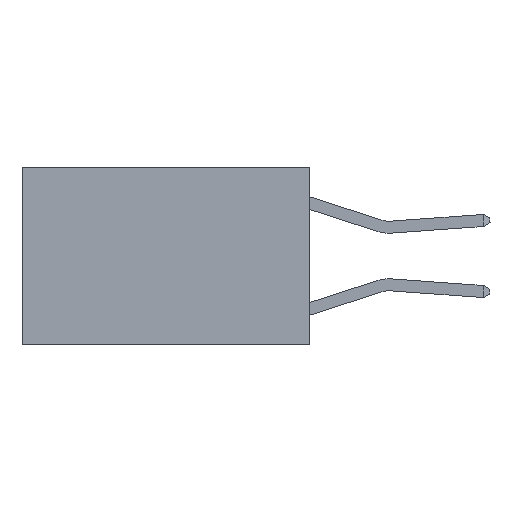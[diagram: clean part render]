
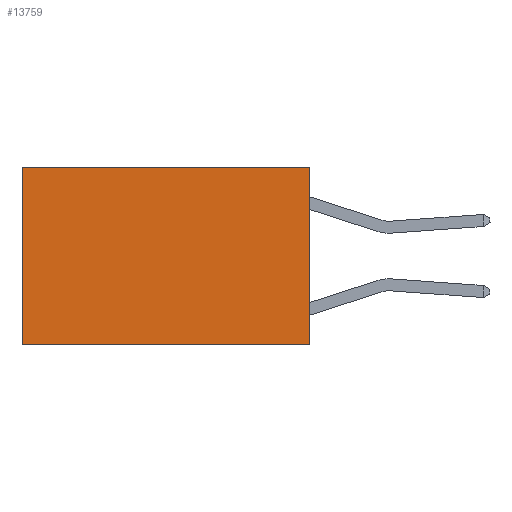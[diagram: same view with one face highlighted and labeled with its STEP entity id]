
A CAD part, left-side view. The second image highlights one B-rep face of the part: STEP entity #13759.
In plain terms, the highlighted planar face has unit normal (-1, 0, 0).
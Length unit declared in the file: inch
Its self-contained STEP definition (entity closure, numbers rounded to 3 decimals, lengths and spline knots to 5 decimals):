
#120 = LINE ( 'NONE', #24694, #15222 ) ;
#196 = CARTESIAN_POINT ( 'NONE',  ( 0.2625, 0., 0. ) ) ;
#549 = VERTEX_POINT ( 'NONE', #26338 ) ;
#1926 = CARTESIAN_POINT ( 'NONE',  ( 0.2625, 0., 0. ) ) ;
#2288 = LINE ( 'NONE', #196, #28103 ) ;
#2440 = CARTESIAN_POINT ( 'NONE',  ( 0.2625, 0., -0.37 ) ) ;
#3439 = EDGE_LOOP ( 'NONE', ( #15402, #12387, #4497, #25152 ) ) ;
#4307 = EDGE_CURVE ( 'NONE', #549, #20545, #120, .T. ) ;
#4382 = EDGE_CURVE ( 'NONE', #549, #28706, #2288, .T. ) ;
#4497 = ORIENTED_EDGE ( 'NONE', *, *, #4382, .F. ) ;
#5279 = VERTEX_POINT ( 'NONE', #22078 ) ;
#8435 = CARTESIAN_POINT ( 'NONE',  ( 0.2625, 0., -0.37 ) ) ;
#10500 = EDGE_CURVE ( 'NONE', #20545, #5279, #24460, .T. ) ;
#10551 = DIRECTION ( 'NONE',  ( 0., 0., -1. ) ) ;
#10690 = FACE_OUTER_BOUND ( 'NONE', #3439, .T. ) ;
#11121 = DIRECTION ( 'NONE',  ( 1., 0., 0. ) ) ;
#11201 = DIRECTION ( 'NONE',  ( 0., 0., -1. ) ) ;
#12387 = ORIENTED_EDGE ( 'NONE', *, *, #16232, .F. ) ;
#13188 = CARTESIAN_POINT ( 'NONE',  ( 0.2625, 0.6, 0. ) ) ;
#13418 = DIRECTION ( 'NONE',  ( 0., 1., 0. ) ) ;
#13571 = DIRECTION ( 'NONE',  ( 0., 1., 0. ) ) ;
#13759 = ADVANCED_FACE ( 'NONE', ( #10690 ), #22103, .F. ) ;
#15222 = VECTOR ( 'NONE', #13571, 39.37008 ) ;
#15402 = ORIENTED_EDGE ( 'NONE', *, *, #10500, .T. ) ;
#15859 = DIRECTION ( 'NONE',  ( 0., 0., -1. ) ) ;
#16232 = EDGE_CURVE ( 'NONE', #28706, #5279, #25274, .T. ) ;
#20545 = VERTEX_POINT ( 'NONE', #27753 ) ;
#20757 = VECTOR ( 'NONE', #13418, 39.37008 ) ;
#22078 = CARTESIAN_POINT ( 'NONE',  ( 0.2625, 0.6, -0.37 ) ) ;
#22103 = PLANE ( 'NONE',  #23994 ) ;
#23449 = VECTOR ( 'NONE', #15859, 39.37008 ) ;
#23994 = AXIS2_PLACEMENT_3D ( 'NONE', #1926, #11121, #10551 ) ;
#24460 = LINE ( 'NONE', #13188, #23449 ) ;
#24694 = CARTESIAN_POINT ( 'NONE',  ( 0.2625, 0., 0. ) ) ;
#25152 = ORIENTED_EDGE ( 'NONE', *, *, #4307, .T. ) ;
#25274 = LINE ( 'NONE', #2440, #20757 ) ;
#26338 = CARTESIAN_POINT ( 'NONE',  ( 0.2625, 0., 0. ) ) ;
#27753 = CARTESIAN_POINT ( 'NONE',  ( 0.2625, 0.6, 0. ) ) ;
#28103 = VECTOR ( 'NONE', #11201, 39.37008 ) ;
#28706 = VERTEX_POINT ( 'NONE', #8435 ) ;
